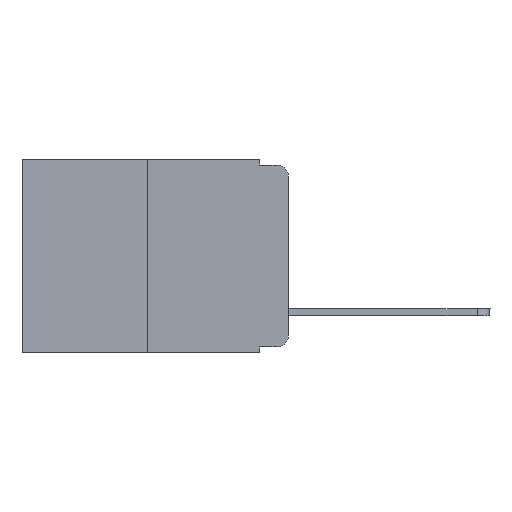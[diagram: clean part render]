
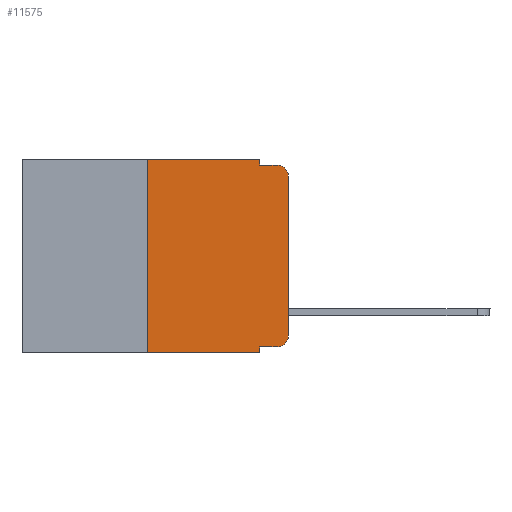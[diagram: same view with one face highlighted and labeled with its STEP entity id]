
A CAD part, left-side view. The second image highlights one B-rep face of the part: STEP entity #11575.
In plain terms, the highlighted planar face has unit normal (-1, 0, 0).
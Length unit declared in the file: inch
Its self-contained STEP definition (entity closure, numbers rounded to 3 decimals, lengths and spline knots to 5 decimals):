
#31 = CARTESIAN_POINT ( 'NONE',  ( 0., 0., -0.313 ) ) ;
#202 = VECTOR ( 'NONE', #12137, 39.37008 ) ;
#521 = ORIENTED_EDGE ( 'NONE', *, *, #21861, .T. ) ;
#1902 = VERTEX_POINT ( 'NONE', #17795 ) ;
#1996 = VERTEX_POINT ( 'NONE', #15528 ) ;
#2234 = CARTESIAN_POINT ( 'NONE',  ( 0., 0.051, -0.01 ) ) ;
#2395 = LINE ( 'NONE', #14650, #18864 ) ;
#2592 = VERTEX_POINT ( 'NONE', #10047 ) ;
#3501 = ORIENTED_EDGE ( 'NONE', *, *, #11289, .T. ) ;
#3917 = DIRECTION ( 'NONE',  ( 0., -1., 0. ) ) ;
#4232 = EDGE_CURVE ( 'NONE', #21484, #7992, #14652, .T. ) ;
#4306 = EDGE_CURVE ( 'NONE', #10048, #2592, #14950, .T. ) ;
#4449 = VECTOR ( 'NONE', #3917, 39.37008 ) ;
#4537 = CIRCLE ( 'NONE', #8075, 0.02 ) ;
#4759 = AXIS2_PLACEMENT_3D ( 'NONE', #13468, #10233, #15531 ) ;
#4987 = CARTESIAN_POINT ( 'NONE',  ( 0., 0.473, 0. ) ) ;
#5062 = EDGE_CURVE ( 'NONE', #12287, #21484, #23039, .T. ) ;
#5174 = VERTEX_POINT ( 'NONE', #8304 ) ;
#5551 = VECTOR ( 'NONE', #7551, 39.37008 ) ;
#6513 = CARTESIAN_POINT ( 'NONE',  ( 0., 0.25, -0.343 ) ) ;
#6643 = VECTOR ( 'NONE', #18707, 39.37008 ) ;
#6876 = ORIENTED_EDGE ( 'NONE', *, *, #18084, .F. ) ;
#6975 = EDGE_CURVE ( 'NONE', #10048, #5174, #8160, .T. ) ;
#7059 = LINE ( 'NONE', #14028, #16724 ) ;
#7490 = VERTEX_POINT ( 'NONE', #31 ) ;
#7551 = DIRECTION ( 'NONE',  ( 0., 0., 1. ) ) ;
#7984 = CIRCLE ( 'NONE', #14470, 0.02 ) ;
#7992 = VERTEX_POINT ( 'NONE', #10776 ) ;
#8075 = AXIS2_PLACEMENT_3D ( 'NONE', #22433, #17189, #13619 ) ;
#8160 = LINE ( 'NONE', #21578, #16953 ) ;
#8304 = CARTESIAN_POINT ( 'NONE',  ( 0., 0.051, -0.343 ) ) ;
#8559 = ORIENTED_EDGE ( 'NONE', *, *, #12612, .F. ) ;
#8588 = DIRECTION ( 'NONE',  ( 0., 0., -1. ) ) ;
#9488 = CARTESIAN_POINT ( 'NONE',  ( 0., 0.25, 0. ) ) ;
#9514 = DIRECTION ( 'NONE',  ( 0., -1., 0. ) ) ;
#9943 = ORIENTED_EDGE ( 'NONE', *, *, #4306, .F. ) ;
#10002 = PLANE ( 'NONE',  #4759 ) ;
#10047 = CARTESIAN_POINT ( 'NONE',  ( 0., 0.25, 0. ) ) ;
#10048 = VERTEX_POINT ( 'NONE', #6513 ) ;
#10212 = CARTESIAN_POINT ( 'NONE',  ( 0., 0.02, -0.333 ) ) ;
#10233 = DIRECTION ( 'NONE',  ( 1., 0., 0. ) ) ;
#10776 = CARTESIAN_POINT ( 'NONE',  ( 0., 0.02, -0.01 ) ) ;
#11078 = VECTOR ( 'NONE', #18934, 39.37008 ) ;
#11289 = EDGE_CURVE ( 'NONE', #1902, #7992, #7984, .T. ) ;
#11376 = ORIENTED_EDGE ( 'NONE', *, *, #11619, .T. ) ;
#11575 = ADVANCED_FACE ( 'NONE', ( #11669 ), #10002, .F. ) ;
#11619 = EDGE_CURVE ( 'NONE', #7490, #1902, #12228, .T. ) ;
#11669 = FACE_OUTER_BOUND ( 'NONE', #15965, .T. ) ;
#12020 = ORIENTED_EDGE ( 'NONE', *, *, #6975, .T. ) ;
#12137 = DIRECTION ( 'NONE',  ( 0., -1., 0. ) ) ;
#12228 = LINE ( 'NONE', #20939, #11078 ) ;
#12237 = VERTEX_POINT ( 'NONE', #10212 ) ;
#12287 = VERTEX_POINT ( 'NONE', #23415 ) ;
#12612 = EDGE_CURVE ( 'NONE', #2592, #12287, #15023, .T. ) ;
#13468 = CARTESIAN_POINT ( 'NONE',  ( 0., 0.473, 0. ) ) ;
#13619 = DIRECTION ( 'NONE',  ( 0., 0., -1. ) ) ;
#14028 = CARTESIAN_POINT ( 'NONE',  ( 0., 0.051, 0. ) ) ;
#14470 = AXIS2_PLACEMENT_3D ( 'NONE', #22800, #20828, #8588 ) ;
#14650 = CARTESIAN_POINT ( 'NONE',  ( 0., 0.051, -0.333 ) ) ;
#14652 = LINE ( 'NONE', #2234, #4449 ) ;
#14950 = LINE ( 'NONE', #9488, #5551 ) ;
#15023 = LINE ( 'NONE', #4987, #202 ) ;
#15045 = ORIENTED_EDGE ( 'NONE', *, *, #5062, .F. ) ;
#15528 = CARTESIAN_POINT ( 'NONE',  ( 0., 0.051, -0.333 ) ) ;
#15531 = DIRECTION ( 'NONE',  ( 0., 0., -1. ) ) ;
#15965 = EDGE_LOOP ( 'NONE', ( #11376, #3501, #20192, #15045, #8559, #9943, #12020, #6876, #521, #16347 ) ) ;
#16347 = ORIENTED_EDGE ( 'NONE', *, *, #18486, .T. ) ;
#16724 = VECTOR ( 'NONE', #17761, 39.37008 ) ;
#16953 = VECTOR ( 'NONE', #17020, 39.37008 ) ;
#17020 = DIRECTION ( 'NONE',  ( 0., -1., 0. ) ) ;
#17189 = DIRECTION ( 'NONE',  ( -1., 0., 0. ) ) ;
#17761 = DIRECTION ( 'NONE',  ( 0., 0., -1. ) ) ;
#17795 = CARTESIAN_POINT ( 'NONE',  ( 0., 0., -0.03 ) ) ;
#18084 = EDGE_CURVE ( 'NONE', #1996, #5174, #7059, .T. ) ;
#18486 = EDGE_CURVE ( 'NONE', #12237, #7490, #4537, .T. ) ;
#18707 = DIRECTION ( 'NONE',  ( 0., 0., -1. ) ) ;
#18864 = VECTOR ( 'NONE', #9514, 39.37008 ) ;
#18934 = DIRECTION ( 'NONE',  ( 0., 0., 1. ) ) ;
#19097 = CARTESIAN_POINT ( 'NONE',  ( 0., 0.051, -0.01 ) ) ;
#20192 = ORIENTED_EDGE ( 'NONE', *, *, #4232, .F. ) ;
#20828 = DIRECTION ( 'NONE',  ( -1., 0., 0. ) ) ;
#20939 = CARTESIAN_POINT ( 'NONE',  ( 0., 0., 0. ) ) ;
#21484 = VERTEX_POINT ( 'NONE', #19097 ) ;
#21578 = CARTESIAN_POINT ( 'NONE',  ( 0., 0.473, -0.343 ) ) ;
#21861 = EDGE_CURVE ( 'NONE', #1996, #12237, #2395, .T. ) ;
#22207 = CARTESIAN_POINT ( 'NONE',  ( 0., 0.051, 0. ) ) ;
#22433 = CARTESIAN_POINT ( 'NONE',  ( 0., 0.02, -0.313 ) ) ;
#22800 = CARTESIAN_POINT ( 'NONE',  ( 0., 0.02, -0.03 ) ) ;
#23039 = LINE ( 'NONE', #22207, #6643 ) ;
#23415 = CARTESIAN_POINT ( 'NONE',  ( 0., 0.051, 0. ) ) ;
